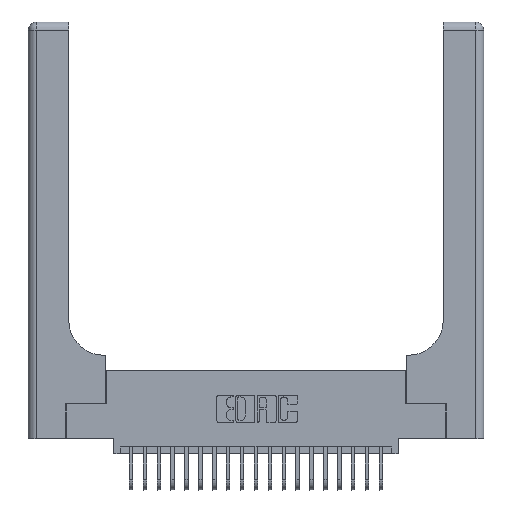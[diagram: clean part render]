
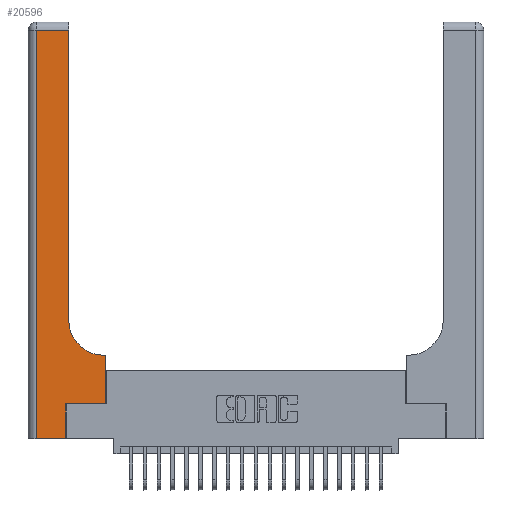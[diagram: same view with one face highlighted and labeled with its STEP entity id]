
A CAD part, top view. The second image highlights one B-rep face of the part: STEP entity #20596.
In plain terms, the highlighted planar face has unit normal (0, 0, 1).
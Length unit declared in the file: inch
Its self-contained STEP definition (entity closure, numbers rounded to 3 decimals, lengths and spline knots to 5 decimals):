
#389 = LINE ( 'NONE', #17466, #10810 ) ;
#874 = LINE ( 'NONE', #3655, #6151 ) ;
#1606 = DIRECTION ( 'NONE',  ( 1., 0., 0. ) ) ;
#1657 = VECTOR ( 'NONE', #1606, 39.37008 ) ;
#1772 = ORIENTED_EDGE ( 'NONE', *, *, #3716, .T. ) ;
#2353 = CARTESIAN_POINT ( 'NONE',  ( 0., 3., 0.37 ) ) ;
#2621 = CARTESIAN_POINT ( 'NONE',  ( 0.5415, 0.6, 0.37 ) ) ;
#3188 = AXIS2_PLACEMENT_3D ( 'NONE', #8349, #21773, #10280 ) ;
#3231 = AXIS2_PLACEMENT_3D ( 'NONE', #2353, #17876, #6325 ) ;
#3542 = CARTESIAN_POINT ( 'NONE',  ( 0.269, 0.25, 0.37 ) ) ;
#3655 = CARTESIAN_POINT ( 'NONE',  ( 0., 2.94, 0.37 ) ) ;
#3716 = EDGE_CURVE ( 'NONE', #19481, #14857, #874, .T. ) ;
#3821 = CARTESIAN_POINT ( 'NONE',  ( 0.2915, 2.94, 0.37 ) ) ;
#4061 = EDGE_CURVE ( 'NONE', #19603, #11622, #14929, .T. ) ;
#4234 = ORIENTED_EDGE ( 'NONE', *, *, #17529, .T. ) ;
#5065 = LINE ( 'NONE', #23304, #18648 ) ;
#5627 = ORIENTED_EDGE ( 'NONE', *, *, #24323, .T. ) ;
#5897 = DIRECTION ( 'NONE',  ( 0., 1., 0. ) ) ;
#6016 = DIRECTION ( 'NONE',  ( 0., 1., 0. ) ) ;
#6151 = VECTOR ( 'NONE', #24728, 39.37008 ) ;
#6325 = DIRECTION ( 'NONE',  ( -1., 0., 0. ) ) ;
#6992 = CIRCLE ( 'NONE', #3188, 0.25 ) ;
#6996 = CARTESIAN_POINT ( 'NONE',  ( 0., 0., 0.37 ) ) ;
#7070 = CARTESIAN_POINT ( 'NONE',  ( 0.06, 0., 0.37 ) ) ;
#7309 = CARTESIAN_POINT ( 'NONE',  ( 0.06, 3., 0.37 ) ) ;
#8349 = CARTESIAN_POINT ( 'NONE',  ( 0.5415, 0.85, 0.37 ) ) ;
#8444 = ORIENTED_EDGE ( 'NONE', *, *, #23736, .T. ) ;
#8445 = ORIENTED_EDGE ( 'NONE', *, *, #11723, .T. ) ;
#9264 = DIRECTION ( 'NONE',  ( 0., -1., 0. ) ) ;
#10280 = DIRECTION ( 'NONE',  ( 1., 0., 0. ) ) ;
#10810 = VECTOR ( 'NONE', #5897, 39.37008 ) ;
#10860 = CARTESIAN_POINT ( 'NONE',  ( 0.5585, 0.6, 0.37 ) ) ;
#11461 = LINE ( 'NONE', #19225, #1657 ) ;
#11622 = VERTEX_POINT ( 'NONE', #10860 ) ;
#11629 = CARTESIAN_POINT ( 'NONE',  ( 0.2915, 0.6, 0.37 ) ) ;
#11723 = EDGE_CURVE ( 'NONE', #14857, #13580, #24671, .T. ) ;
#12312 = CARTESIAN_POINT ( 'NONE',  ( 0.5585, 0.25, 0.37 ) ) ;
#13580 = VERTEX_POINT ( 'NONE', #7070 ) ;
#13753 = VERTEX_POINT ( 'NONE', #3542 ) ;
#13770 = EDGE_CURVE ( 'NONE', #13753, #19603, #11461, .T. ) ;
#13943 = CARTESIAN_POINT ( 'NONE',  ( 0.5585, 0.25, 0.37 ) ) ;
#14053 = PLANE ( 'NONE',  #3231 ) ;
#14279 = DIRECTION ( 'NONE',  ( 0., 1., 0. ) ) ;
#14596 = VECTOR ( 'NONE', #9264, 39.37008 ) ;
#14857 = VERTEX_POINT ( 'NONE', #17798 ) ;
#14929 = LINE ( 'NONE', #12312, #15535 ) ;
#14994 = VERTEX_POINT ( 'NONE', #2621 ) ;
#15525 = DIRECTION ( 'NONE',  ( -1., 0., 0. ) ) ;
#15535 = VECTOR ( 'NONE', #14279, 39.37008 ) ;
#15809 = CARTESIAN_POINT ( 'NONE',  ( 0.269, 0., 0.37 ) ) ;
#15915 = ORIENTED_EDGE ( 'NONE', *, *, #13770, .T. ) ;
#16251 = FACE_OUTER_BOUND ( 'NONE', #19329, .T. ) ;
#17177 = VECTOR ( 'NONE', #15525, 39.37008 ) ;
#17193 = ORIENTED_EDGE ( 'NONE', *, *, #17901, .T. ) ;
#17342 = ORIENTED_EDGE ( 'NONE', *, *, #4061, .T. ) ;
#17466 = CARTESIAN_POINT ( 'NONE',  ( 0.269, 0., 0.37 ) ) ;
#17529 = EDGE_CURVE ( 'NONE', #13580, #19079, #20591, .T. ) ;
#17656 = VERTEX_POINT ( 'NONE', #24713 ) ;
#17798 = CARTESIAN_POINT ( 'NONE',  ( 0.06, 2.94, 0.37 ) ) ;
#17876 = DIRECTION ( 'NONE',  ( 0., 0., -1. ) ) ;
#17901 = EDGE_CURVE ( 'NONE', #14994, #17656, #6992, .T. ) ;
#18632 = DIRECTION ( 'NONE',  ( 1., 0., 0. ) ) ;
#18648 = VECTOR ( 'NONE', #6016, 39.37008 ) ;
#19079 = VERTEX_POINT ( 'NONE', #15809 ) ;
#19208 = ORIENTED_EDGE ( 'NONE', *, *, #23140, .T. ) ;
#19225 = CARTESIAN_POINT ( 'NONE',  ( 0.269, 0.25, 0.37 ) ) ;
#19329 = EDGE_LOOP ( 'NONE', ( #8444, #1772, #8445, #4234, #5627, #15915, #17342, #19208, #17193 ) ) ;
#19405 = VECTOR ( 'NONE', #18632, 39.37008 ) ;
#19481 = VERTEX_POINT ( 'NONE', #3821 ) ;
#19603 = VERTEX_POINT ( 'NONE', #13943 ) ;
#20591 = LINE ( 'NONE', #6996, #19405 ) ;
#20596 = ADVANCED_FACE ( 'NONE', ( #16251 ), #14053, .F. ) ;
#21657 = LINE ( 'NONE', #11629, #17177 ) ;
#21773 = DIRECTION ( 'NONE',  ( 0., 0., -1. ) ) ;
#23140 = EDGE_CURVE ( 'NONE', #11622, #14994, #21657, .T. ) ;
#23304 = CARTESIAN_POINT ( 'NONE',  ( 0.2915, 3., 0.37 ) ) ;
#23736 = EDGE_CURVE ( 'NONE', #17656, #19481, #5065, .T. ) ;
#24323 = EDGE_CURVE ( 'NONE', #19079, #13753, #389, .T. ) ;
#24671 = LINE ( 'NONE', #7309, #14596 ) ;
#24713 = CARTESIAN_POINT ( 'NONE',  ( 0.2915, 0.85, 0.37 ) ) ;
#24728 = DIRECTION ( 'NONE',  ( -1., 0., 0. ) ) ;
